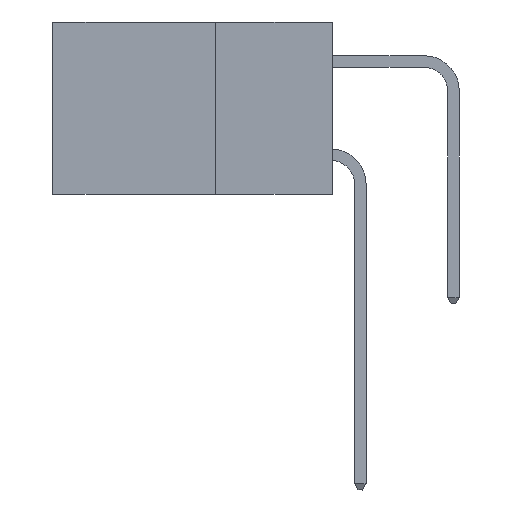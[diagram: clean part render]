
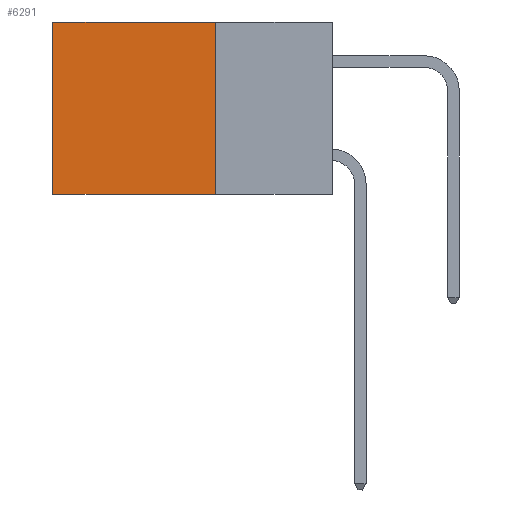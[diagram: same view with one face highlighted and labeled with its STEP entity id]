
A CAD part, left-side view. The second image highlights one B-rep face of the part: STEP entity #6291.
In plain terms, the highlighted planar face has unit normal (-1, 0, 0).
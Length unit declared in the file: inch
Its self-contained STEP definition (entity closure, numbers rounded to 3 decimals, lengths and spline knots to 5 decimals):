
#13 = LINE ( 'NONE', #199, #5358 ) ;
#58 = DIRECTION ( 'NONE',  ( 0., 0., -1. ) ) ;
#96 = ORIENTED_EDGE ( 'NONE', *, *, #1735, .F. ) ;
#175 = AXIS2_PLACEMENT_3D ( 'NONE', #6790, #6747, #3477 ) ;
#199 = CARTESIAN_POINT ( 'NONE',  ( 0.298, 0.25, -0.37 ) ) ;
#1310 = DIRECTION ( 'NONE',  ( 0., 1., 0. ) ) ;
#1735 = EDGE_CURVE ( 'NONE', #4780, #10042, #13, .T. ) ;
#3477 = DIRECTION ( 'NONE',  ( 0., 0., -1. ) ) ;
#4113 = LINE ( 'NONE', #11065, #13185 ) ;
#4466 = PLANE ( 'NONE',  #175 ) ;
#4780 = VERTEX_POINT ( 'NONE', #11478 ) ;
#5015 = CARTESIAN_POINT ( 'NONE',  ( 0.298, 0.25, 0. ) ) ;
#5358 = VECTOR ( 'NONE', #1310, 39.37008 ) ;
#5367 = EDGE_LOOP ( 'NONE', ( #7524, #96, #6805, #13138 ) ) ;
#5434 = VERTEX_POINT ( 'NONE', #7001 ) ;
#5794 = CARTESIAN_POINT ( 'NONE',  ( 0.298, 0.25, 0. ) ) ;
#5825 = FACE_OUTER_BOUND ( 'NONE', #5367, .T. ) ;
#5835 = VECTOR ( 'NONE', #13645, 39.37008 ) ;
#6291 = ADVANCED_FACE ( 'NONE', ( #5825 ), #4466, .F. ) ;
#6465 = VERTEX_POINT ( 'NONE', #5015 ) ;
#6747 = DIRECTION ( 'NONE',  ( 1., 0., 0. ) ) ;
#6790 = CARTESIAN_POINT ( 'NONE',  ( 0.298, 0.25, 0. ) ) ;
#6805 = ORIENTED_EDGE ( 'NONE', *, *, #12478, .F. ) ;
#7001 = CARTESIAN_POINT ( 'NONE',  ( 0.298, 0.6, 0. ) ) ;
#7441 = EDGE_CURVE ( 'NONE', #5434, #10042, #4113, .T. ) ;
#7524 = ORIENTED_EDGE ( 'NONE', *, *, #7441, .T. ) ;
#8193 = CARTESIAN_POINT ( 'NONE',  ( 0.298, 0.6, -0.37 ) ) ;
#9087 = EDGE_CURVE ( 'NONE', #6465, #5434, #10232, .T. ) ;
#10042 = VERTEX_POINT ( 'NONE', #8193 ) ;
#10232 = LINE ( 'NONE', #13399, #13990 ) ;
#10276 = DIRECTION ( 'NONE',  ( 0., 1., 0. ) ) ;
#10533 = LINE ( 'NONE', #5794, #5835 ) ;
#11065 = CARTESIAN_POINT ( 'NONE',  ( 0.298, 0.6, 0. ) ) ;
#11478 = CARTESIAN_POINT ( 'NONE',  ( 0.298, 0.25, -0.37 ) ) ;
#12478 = EDGE_CURVE ( 'NONE', #6465, #4780, #10533, .T. ) ;
#13138 = ORIENTED_EDGE ( 'NONE', *, *, #9087, .T. ) ;
#13185 = VECTOR ( 'NONE', #58, 39.37008 ) ;
#13399 = CARTESIAN_POINT ( 'NONE',  ( 0.298, 0.25, 0. ) ) ;
#13645 = DIRECTION ( 'NONE',  ( 0., 0., -1. ) ) ;
#13990 = VECTOR ( 'NONE', #10276, 39.37008 ) ;
